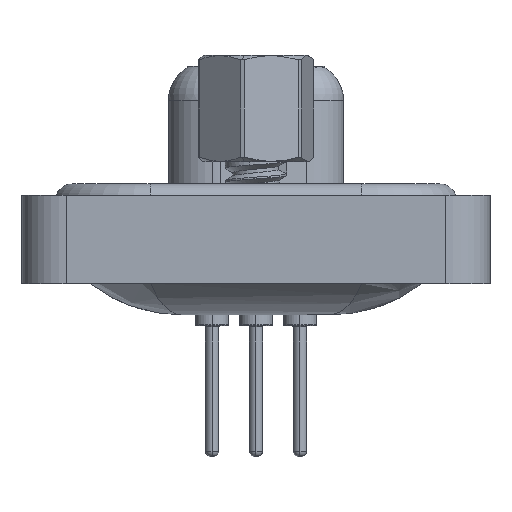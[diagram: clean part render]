
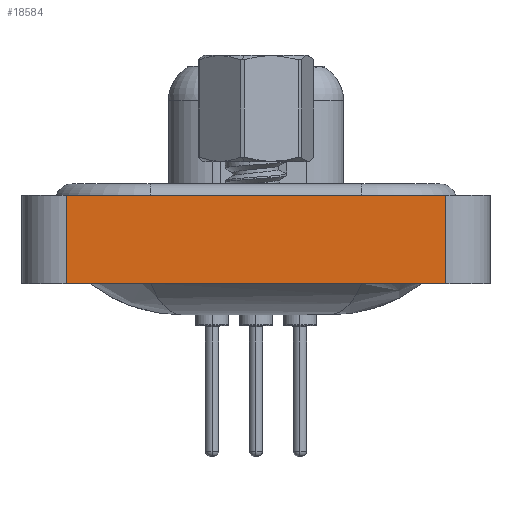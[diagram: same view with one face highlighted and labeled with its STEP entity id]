
A CAD part, left-side view. The second image highlights one B-rep face of the part: STEP entity #18584.
In plain terms, the highlighted planar face has unit normal (-1, 0, 0).
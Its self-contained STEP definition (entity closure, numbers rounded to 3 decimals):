
#4486 = VECTOR ( 'NONE', #14567, 1000. ) ;
#4657 = CARTESIAN_POINT ( 'NONE',  ( -7.285, -8.55, -3.6 ) ) ;
#4724 = ORIENTED_EDGE ( 'NONE', *, *, #23370, .T. ) ;
#4819 = CARTESIAN_POINT ( 'NONE',  ( -7.285, -8.55, 0.4 ) ) ;
#5065 = AXIS2_PLACEMENT_3D ( 'NONE', #23944, #16805, #18811 ) ;
#5160 = EDGE_CURVE ( 'NONE', #17430, #29424, #17162, .T. ) ;
#8486 = CARTESIAN_POINT ( 'NONE',  ( -7.285, 8.55, 0.4 ) ) ;
#10912 = DIRECTION ( 'NONE',  ( 0., 0., 1. ) ) ;
#11375 = CARTESIAN_POINT ( 'NONE',  ( -7.285, -8.55, -3.6 ) ) ;
#11472 = VERTEX_POINT ( 'NONE', #17875 ) ;
#12391 = ORIENTED_EDGE ( 'NONE', *, *, #30020, .T. ) ;
#12758 = CARTESIAN_POINT ( 'NONE',  ( -7.285, 8.55, -3.6 ) ) ;
#13529 = ORIENTED_EDGE ( 'NONE', *, *, #27307, .F. ) ;
#14567 = DIRECTION ( 'NONE',  ( 0., -1., 0. ) ) ;
#14846 = DIRECTION ( 'NONE',  ( 0., 0., 1. ) ) ;
#16805 = DIRECTION ( 'NONE',  ( -1., 0., 0. ) ) ;
#17021 = VECTOR ( 'NONE', #14846, 1000. ) ;
#17162 = LINE ( 'NONE', #23983, #17021 ) ;
#17430 = VERTEX_POINT ( 'NONE', #12758 ) ;
#17556 = ORIENTED_EDGE ( 'NONE', *, *, #5160, .F. ) ;
#17589 = VERTEX_POINT ( 'NONE', #4657 ) ;
#17875 = CARTESIAN_POINT ( 'NONE',  ( -7.285, -8.55, 0.4 ) ) ;
#18336 = LINE ( 'NONE', #11375, #24333 ) ;
#18584 = ADVANCED_FACE ( 'NONE', ( #19275 ), #21776, .T. ) ;
#18811 = DIRECTION ( 'NONE',  ( 0., 0., 1. ) ) ;
#19275 = FACE_OUTER_BOUND ( 'NONE', #24641, .T. ) ;
#21536 = LINE ( 'NONE', #4819, #4486 ) ;
#21776 = PLANE ( 'NONE',  #5065 ) ;
#23229 = DIRECTION ( 'NONE',  ( 0., -1., 0. ) ) ;
#23370 = EDGE_CURVE ( 'NONE', #17430, #17589, #30018, .T. ) ;
#23944 = CARTESIAN_POINT ( 'NONE',  ( -7.285, -8.55, -3.6 ) ) ;
#23983 = CARTESIAN_POINT ( 'NONE',  ( -7.285, 8.55, -3.6 ) ) ;
#24333 = VECTOR ( 'NONE', #10912, 1000. ) ;
#24641 = EDGE_LOOP ( 'NONE', ( #12391, #13529, #17556, #4724 ) ) ;
#25534 = CARTESIAN_POINT ( 'NONE',  ( -7.285, -8.55, -3.6 ) ) ;
#27307 = EDGE_CURVE ( 'NONE', #29424, #11472, #21536, .T. ) ;
#29424 = VERTEX_POINT ( 'NONE', #8486 ) ;
#30008 = VECTOR ( 'NONE', #23229, 1000. ) ;
#30018 = LINE ( 'NONE', #25534, #30008 ) ;
#30020 = EDGE_CURVE ( 'NONE', #17589, #11472, #18336, .T. ) ;
